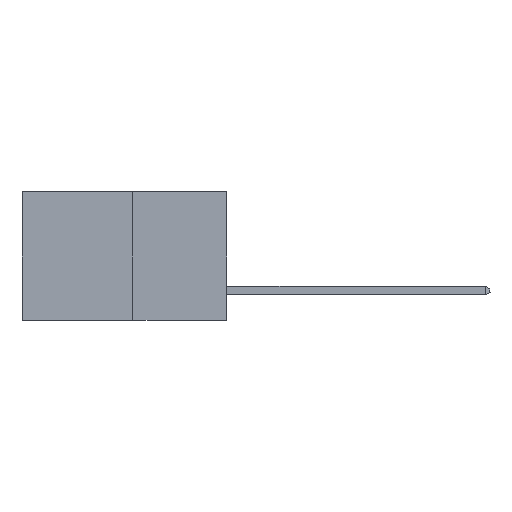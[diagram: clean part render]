
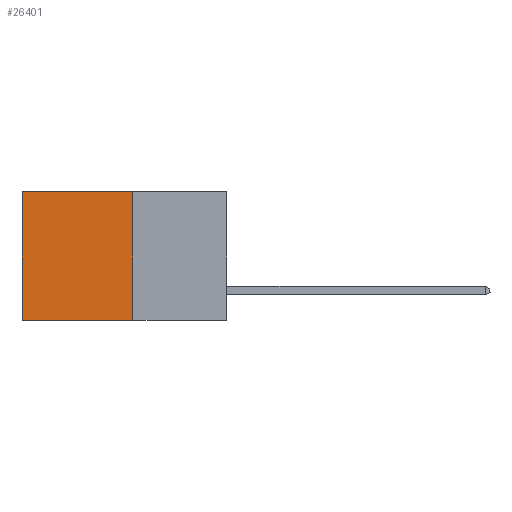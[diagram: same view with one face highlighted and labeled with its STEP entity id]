
A CAD part, left-side view. The second image highlights one B-rep face of the part: STEP entity #26401.
In plain terms, the highlighted planar face has unit normal (-1, 0, 0).
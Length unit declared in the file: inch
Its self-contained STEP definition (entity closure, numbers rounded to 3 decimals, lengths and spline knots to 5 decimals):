
#224 = EDGE_CURVE ( 'NONE', #22520, #14817, #2093, .T. ) ;
#984 = CARTESIAN_POINT ( 'NONE',  ( 0.277, 0.27, 0. ) ) ;
#1056 = LINE ( 'NONE', #14325, #19900 ) ;
#2093 = LINE ( 'NONE', #30974, #28151 ) ;
#2197 = ORIENTED_EDGE ( 'NONE', *, *, #224, .T. ) ;
#2843 = ORIENTED_EDGE ( 'NONE', *, *, #30924, .F. ) ;
#3122 = DIRECTION ( 'NONE',  ( 0., 0., -1. ) ) ;
#3991 = VERTEX_POINT ( 'NONE', #21834 ) ;
#4798 = CARTESIAN_POINT ( 'NONE',  ( 0.277, 0.59, -0.37 ) ) ;
#4922 = VECTOR ( 'NONE', #3122, 39.37008 ) ;
#5883 = CARTESIAN_POINT ( 'NONE',  ( 0.277, 0.59, -0.37 ) ) ;
#6709 = VECTOR ( 'NONE', #27851, 39.37008 ) ;
#7137 = CARTESIAN_POINT ( 'NONE',  ( 0.277, 0.27, -0.37 ) ) ;
#8677 = FACE_OUTER_BOUND ( 'NONE', #11607, .T. ) ;
#9622 = PLANE ( 'NONE',  #13229 ) ;
#9900 = ORIENTED_EDGE ( 'NONE', *, *, #14181, .F. ) ;
#11469 = LINE ( 'NONE', #22690, #4922 ) ;
#11607 = EDGE_LOOP ( 'NONE', ( #28058, #9900, #2843, #2197 ) ) ;
#13229 = AXIS2_PLACEMENT_3D ( 'NONE', #7137, #29129, #14605 ) ;
#13375 = VERTEX_POINT ( 'NONE', #4798 ) ;
#14181 = EDGE_CURVE ( 'NONE', #3991, #13375, #1056, .T. ) ;
#14325 = CARTESIAN_POINT ( 'NONE',  ( 0.277, 0.27, -0.37 ) ) ;
#14441 = DIRECTION ( 'NONE',  ( 0., 1., 0. ) ) ;
#14605 = DIRECTION ( 'NONE',  ( 0., 0., -1. ) ) ;
#14817 = VERTEX_POINT ( 'NONE', #19274 ) ;
#15913 = EDGE_CURVE ( 'NONE', #14817, #13375, #19783, .T. ) ;
#19274 = CARTESIAN_POINT ( 'NONE',  ( 0.277, 0.59, 0. ) ) ;
#19783 = LINE ( 'NONE', #5883, #6709 ) ;
#19900 = VECTOR ( 'NONE', #14441, 39.37008 ) ;
#21834 = CARTESIAN_POINT ( 'NONE',  ( 0.277, 0.27, -0.37 ) ) ;
#22520 = VERTEX_POINT ( 'NONE', #984 ) ;
#22690 = CARTESIAN_POINT ( 'NONE',  ( 0.277, 0.27, -0.37 ) ) ;
#26401 = ADVANCED_FACE ( 'NONE', ( #8677 ), #9622, .F. ) ;
#27851 = DIRECTION ( 'NONE',  ( 0., 0., -1. ) ) ;
#28058 = ORIENTED_EDGE ( 'NONE', *, *, #15913, .T. ) ;
#28151 = VECTOR ( 'NONE', #30772, 39.37008 ) ;
#29129 = DIRECTION ( 'NONE',  ( 1., 0., 0. ) ) ;
#30772 = DIRECTION ( 'NONE',  ( 0., 1., 0. ) ) ;
#30924 = EDGE_CURVE ( 'NONE', #22520, #3991, #11469, .T. ) ;
#30974 = CARTESIAN_POINT ( 'NONE',  ( 0.277, 0.27, 0. ) ) ;
